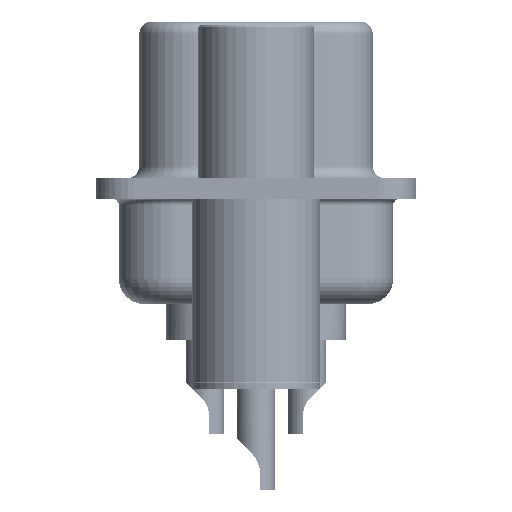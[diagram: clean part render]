
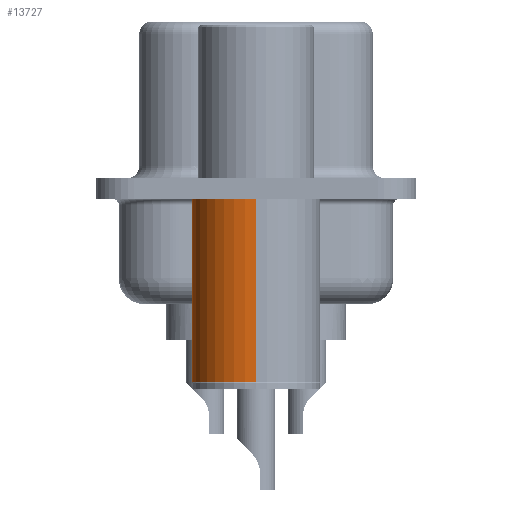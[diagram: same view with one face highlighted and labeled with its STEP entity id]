
A CAD part, left-side view. The second image highlights one B-rep face of the part: STEP entity #13727.
In plain terms, the highlighted cylindrical face has radius 2.5 mm (diameter 5 mm), a partial arc.
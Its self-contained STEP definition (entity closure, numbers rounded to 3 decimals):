
#767 = AXIS2_PLACEMENT_3D ( 'NONE', #14115, #16937, #19661 ) ;
#2512 = EDGE_CURVE ( 'NONE', #10089, #25538, #3374, .T. ) ;
#2589 = CARTESIAN_POINT ( 'NONE',  ( 0., 0., -0.4 ) ) ;
#3374 = CIRCLE ( 'NONE', #18646, 2.5 ) ;
#3710 = ORIENTED_EDGE ( 'NONE', *, *, #30336, .F. ) ;
#3812 = CIRCLE ( 'NONE', #21713, 2.5 ) ;
#5187 = LINE ( 'NONE', #21145, #24858 ) ;
#5316 = DIRECTION ( 'NONE',  ( 1., 0., 0. ) ) ;
#7033 = DIRECTION ( 'NONE',  ( 0., 0., 1. ) ) ;
#8105 = ORIENTED_EDGE ( 'NONE', *, *, #10170, .F. ) ;
#8209 = CARTESIAN_POINT ( 'NONE',  ( 0., 0., -7.525 ) ) ;
#9046 = VERTEX_POINT ( 'NONE', #27494 ) ;
#10089 = VERTEX_POINT ( 'NONE', #23401 ) ;
#10170 = EDGE_CURVE ( 'NONE', #10089, #9046, #26844, .T. ) ;
#10506 = DIRECTION ( 'NONE',  ( 0., 0., 1. ) ) ;
#11809 = CYLINDRICAL_SURFACE ( 'NONE', #767, 2.5 ) ;
#12310 = DIRECTION ( 'NONE',  ( 1., 0., 0. ) ) ;
#13727 = ADVANCED_FACE ( 'NONE', ( #18946 ), #11809, .T. ) ;
#13757 = CARTESIAN_POINT ( 'NONE',  ( -2.5, 0., -7.525 ) ) ;
#14115 = CARTESIAN_POINT ( 'NONE',  ( 0., 0., 0.581 ) ) ;
#15384 = VERTEX_POINT ( 'NONE', #23411 ) ;
#15523 = EDGE_LOOP ( 'NONE', ( #22840, #20156, #3710, #8105 ) ) ;
#16937 = DIRECTION ( 'NONE',  ( 0., 0., 1. ) ) ;
#18646 = AXIS2_PLACEMENT_3D ( 'NONE', #8209, #7033, #12310 ) ;
#18946 = FACE_OUTER_BOUND ( 'NONE', #15523, .T. ) ;
#19661 = DIRECTION ( 'NONE',  ( 1., 0., 0. ) ) ;
#20156 = ORIENTED_EDGE ( 'NONE', *, *, #28971, .T. ) ;
#21145 = CARTESIAN_POINT ( 'NONE',  ( -2.5, 0., 0.581 ) ) ;
#21439 = DIRECTION ( 'NONE',  ( 0., 0., 1. ) ) ;
#21713 = AXIS2_PLACEMENT_3D ( 'NONE', #2589, #21439, #5316 ) ;
#22840 = ORIENTED_EDGE ( 'NONE', *, *, #2512, .T. ) ;
#23401 = CARTESIAN_POINT ( 'NONE',  ( 2.5, 0., -7.525 ) ) ;
#23411 = CARTESIAN_POINT ( 'NONE',  ( -2.5, 0., -0.4 ) ) ;
#24858 = VECTOR ( 'NONE', #10506, 1000. ) ;
#25538 = VERTEX_POINT ( 'NONE', #13757 ) ;
#26119 = DIRECTION ( 'NONE',  ( 0., 0., 1. ) ) ;
#26844 = LINE ( 'NONE', #34007, #33055 ) ;
#27494 = CARTESIAN_POINT ( 'NONE',  ( 2.5, 0., -0.4 ) ) ;
#28971 = EDGE_CURVE ( 'NONE', #25538, #15384, #5187, .T. ) ;
#30336 = EDGE_CURVE ( 'NONE', #9046, #15384, #3812, .T. ) ;
#33055 = VECTOR ( 'NONE', #26119, 1000. ) ;
#34007 = CARTESIAN_POINT ( 'NONE',  ( 2.5, 0., 0.581 ) ) ;
